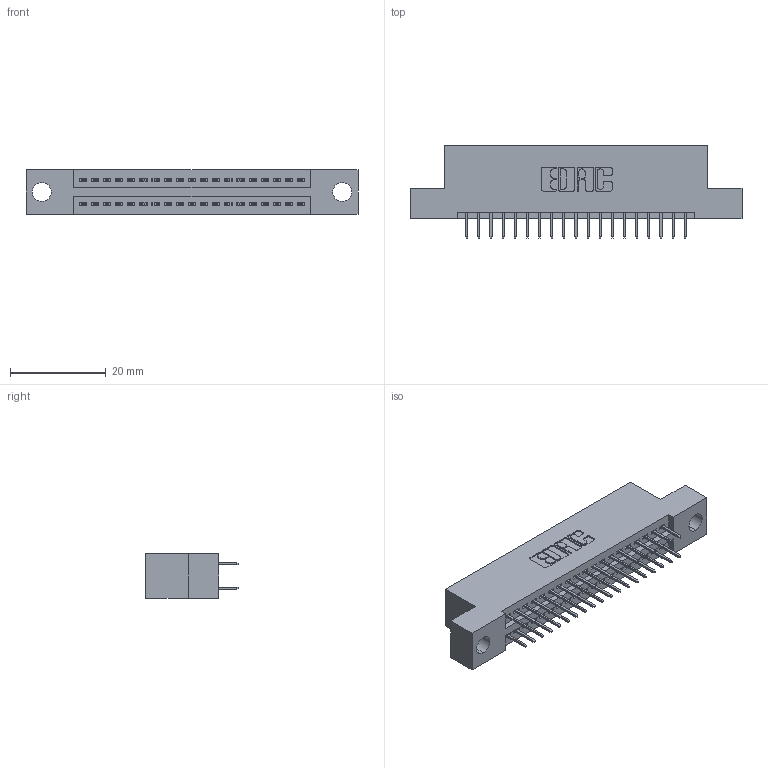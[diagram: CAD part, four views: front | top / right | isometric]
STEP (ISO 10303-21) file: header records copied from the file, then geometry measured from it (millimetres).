
FILE_DESCRIPTION (( 'STEP AP203' ), '1' );
FILE_NAME ('345-038-524-204.STEP', '2021-05-20T00:44:32', ( '' ), ( '' ), 'SwSTEP 2.0', 'SolidWorks 2020', '' );
FILE_SCHEMA (( 'CONFIG_CONTROL_DESIGN' ));
Length unit declared in the file: inch
Products named in the file (3): 345-292-001_345-293-124; 345-038-524-204; 345 Part_Flush Mounting Lugs - 0.156 Dia-TI
Assembly tree (39 placements, depth 2):
  345-038-524-204
    345 Part_Flush Mounting Lugs - 0.156 Dia-TI
    345-292-001_345-293-124  x38
Bounding box: 69.47 x 19.35 x 9.4 mm (x, y, z)
Volume: 6371.3 mm3; surface area: 8672.2 mm2
Topology: 39 solids, 39 shells, 2192 faces, 6191 edges, 3974 vertices
Faces by surface type: plane 1576, cylinder 616
Entity records: 18497 total; most frequent: CARTESIAN_POINT 3126, ORIENTED_EDGE 3058, DIRECTION 2785, EDGE_CURVE 1529, LINE 1325, VECTOR 1325, VERTEX_POINT 1014, AXIS2_PLACEMENT_3D 730
